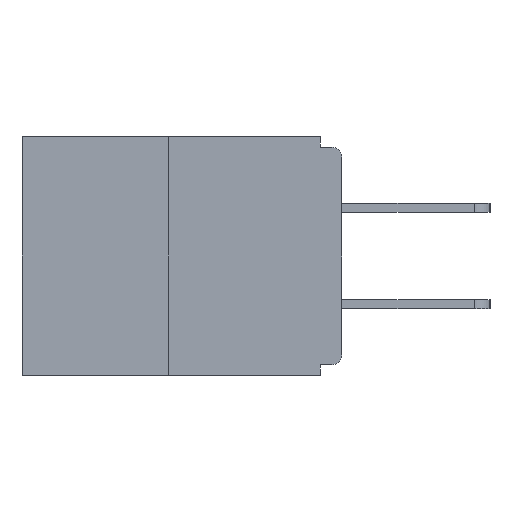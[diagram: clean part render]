
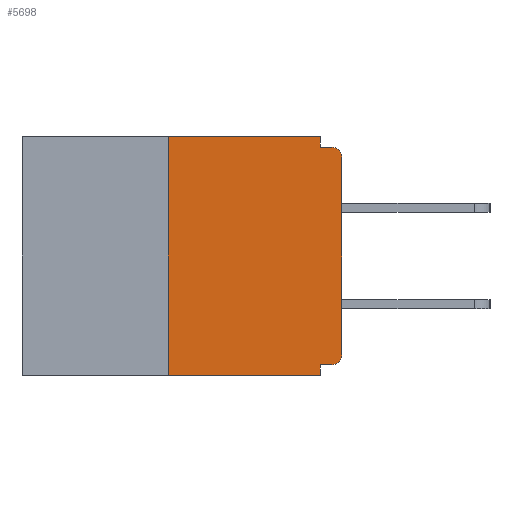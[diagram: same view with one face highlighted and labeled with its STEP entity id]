
A CAD part, left-side view. The second image highlights one B-rep face of the part: STEP entity #5698.
In plain terms, the highlighted planar face has unit normal (-1, 0, 0).
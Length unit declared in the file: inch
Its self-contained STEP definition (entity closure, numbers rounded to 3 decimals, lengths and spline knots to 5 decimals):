
#216 = EDGE_CURVE ( 'NONE', #15936, #7112, #509, .T. ) ;
#248 = LINE ( 'NONE', #10143, #14799 ) ;
#308 = ORIENTED_EDGE ( 'NONE', *, *, #7261, .F. ) ;
#509 = LINE ( 'NONE', #12860, #3932 ) ;
#842 = CARTESIAN_POINT ( 'NONE',  ( 0., 0., -0.328 ) ) ;
#1045 = CARTESIAN_POINT ( 'NONE',  ( 0., 0.031, -0.015 ) ) ;
#1249 = DIRECTION ( 'NONE',  ( 1., 0., 0. ) ) ;
#1310 = AXIS2_PLACEMENT_3D ( 'NONE', #16571, #11235, #15291 ) ;
#1340 = EDGE_LOOP ( 'NONE', ( #10820, #16333, #9954, #6503, #308, #12180, #6165, #7404, #17594, #8028 ) ) ;
#1341 = PLANE ( 'NONE',  #3273 ) ;
#1523 = EDGE_CURVE ( 'NONE', #9903, #10534, #248, .T. ) ;
#1557 = LINE ( 'NONE', #13968, #10172 ) ;
#1688 = LINE ( 'NONE', #14015, #9196 ) ;
#2041 = CARTESIAN_POINT ( 'NONE',  ( 0., 0.015, -0.328 ) ) ;
#2292 = CARTESIAN_POINT ( 'NONE',  ( 0., 0., -0.03 ) ) ;
#2333 = EDGE_CURVE ( 'NONE', #14683, #17802, #9135, .T. ) ;
#2402 = VERTEX_POINT ( 'NONE', #2791 ) ;
#2473 = DIRECTION ( 'NONE',  ( 0., 1., 0. ) ) ;
#2717 = EDGE_CURVE ( 'NONE', #6526, #2402, #1688, .T. ) ;
#2791 = CARTESIAN_POINT ( 'NONE',  ( 0., 0.031, 0. ) ) ;
#2970 = DIRECTION ( 'NONE',  ( 0., -1., 0. ) ) ;
#3224 = EDGE_CURVE ( 'NONE', #6011, #7112, #15330, .T. ) ;
#3273 = AXIS2_PLACEMENT_3D ( 'NONE', #10781, #1249, #9414 ) ;
#3932 = VECTOR ( 'NONE', #2970, 39.37008 ) ;
#4334 = CARTESIAN_POINT ( 'NONE',  ( 0., 0.25, 0. ) ) ;
#5257 = VECTOR ( 'NONE', #14759, 39.37008 ) ;
#5698 = ADVANCED_FACE ( 'NONE', ( #12320 ), #1341, .F. ) ;
#6011 = VERTEX_POINT ( 'NONE', #6547 ) ;
#6165 = ORIENTED_EDGE ( 'NONE', *, *, #7522, .T. ) ;
#6370 = LINE ( 'NONE', #842, #9328 ) ;
#6503 = ORIENTED_EDGE ( 'NONE', *, *, #3224, .F. ) ;
#6526 = VERTEX_POINT ( 'NONE', #4334 ) ;
#6547 = CARTESIAN_POINT ( 'NONE',  ( 0., 0.031, -0.328 ) ) ;
#6829 = CARTESIAN_POINT ( 'NONE',  ( 0., 0.031, -0.343 ) ) ;
#7112 = VERTEX_POINT ( 'NONE', #13197 ) ;
#7261 = EDGE_CURVE ( 'NONE', #14683, #6011, #6370, .T. ) ;
#7404 = ORIENTED_EDGE ( 'NONE', *, *, #12833, .T. ) ;
#7458 = CARTESIAN_POINT ( 'NONE',  ( 0., 0., 0. ) ) ;
#7522 = EDGE_CURVE ( 'NONE', #17802, #17340, #10614, .T. ) ;
#7914 = CARTESIAN_POINT ( 'NONE',  ( 0., 0.031, 0. ) ) ;
#8028 = ORIENTED_EDGE ( 'NONE', *, *, #10274, .F. ) ;
#8495 = DIRECTION ( 'NONE',  ( 0., -1., 0. ) ) ;
#9135 = CIRCLE ( 'NONE', #1310, 0.015 ) ;
#9196 = VECTOR ( 'NONE', #8495, 39.37008 ) ;
#9328 = VECTOR ( 'NONE', #2473, 39.37008 ) ;
#9411 = CARTESIAN_POINT ( 'NONE',  ( 0., 0.015, -0.015 ) ) ;
#9414 = DIRECTION ( 'NONE',  ( 0., 0., -1. ) ) ;
#9874 = CARTESIAN_POINT ( 'NONE',  ( 0., 0.015, -0.03 ) ) ;
#9903 = VERTEX_POINT ( 'NONE', #1045 ) ;
#9954 = ORIENTED_EDGE ( 'NONE', *, *, #216, .T. ) ;
#10143 = CARTESIAN_POINT ( 'NONE',  ( 0., 0., -0.015 ) ) ;
#10145 = AXIS2_PLACEMENT_3D ( 'NONE', #9874, #15030, #10973 ) ;
#10172 = VECTOR ( 'NONE', #12527, 39.37008 ) ;
#10235 = DIRECTION ( 'NONE',  ( 0., -1., 0. ) ) ;
#10274 = EDGE_CURVE ( 'NONE', #2402, #9903, #12169, .T. ) ;
#10534 = VERTEX_POINT ( 'NONE', #9411 ) ;
#10614 = LINE ( 'NONE', #7458, #5257 ) ;
#10727 = DIRECTION ( 'NONE',  ( 0., 0., -1. ) ) ;
#10781 = CARTESIAN_POINT ( 'NONE',  ( 0., 0.46, 0. ) ) ;
#10820 = ORIENTED_EDGE ( 'NONE', *, *, #2717, .F. ) ;
#10973 = DIRECTION ( 'NONE',  ( 0., 0., -1. ) ) ;
#11010 = CIRCLE ( 'NONE', #10145, 0.015 ) ;
#11235 = DIRECTION ( 'NONE',  ( -1., 0., 0. ) ) ;
#12169 = LINE ( 'NONE', #7914, #14970 ) ;
#12180 = ORIENTED_EDGE ( 'NONE', *, *, #2333, .T. ) ;
#12320 = FACE_OUTER_BOUND ( 'NONE', #1340, .T. ) ;
#12527 = DIRECTION ( 'NONE',  ( 0., 0., 1. ) ) ;
#12833 = EDGE_CURVE ( 'NONE', #17340, #10534, #11010, .T. ) ;
#12860 = CARTESIAN_POINT ( 'NONE',  ( 0., 0.46, -0.343 ) ) ;
#13197 = CARTESIAN_POINT ( 'NONE',  ( 0., 0.031, -0.343 ) ) ;
#13692 = EDGE_CURVE ( 'NONE', #15936, #6526, #1557, .T. ) ;
#13968 = CARTESIAN_POINT ( 'NONE',  ( 0., 0.25, 0. ) ) ;
#14015 = CARTESIAN_POINT ( 'NONE',  ( 0., 0.46, 0. ) ) ;
#14683 = VERTEX_POINT ( 'NONE', #2041 ) ;
#14759 = DIRECTION ( 'NONE',  ( 0., 0., 1. ) ) ;
#14799 = VECTOR ( 'NONE', #10235, 39.37008 ) ;
#14970 = VECTOR ( 'NONE', #10727, 39.37008 ) ;
#15030 = DIRECTION ( 'NONE',  ( -1., 0., 0. ) ) ;
#15073 = VECTOR ( 'NONE', #16801, 39.37008 ) ;
#15291 = DIRECTION ( 'NONE',  ( 0., 0., -1. ) ) ;
#15330 = LINE ( 'NONE', #6829, #15073 ) ;
#15571 = CARTESIAN_POINT ( 'NONE',  ( 0., 0.25, -0.343 ) ) ;
#15936 = VERTEX_POINT ( 'NONE', #15571 ) ;
#16333 = ORIENTED_EDGE ( 'NONE', *, *, #13692, .F. ) ;
#16571 = CARTESIAN_POINT ( 'NONE',  ( 0., 0.015, -0.313 ) ) ;
#16801 = DIRECTION ( 'NONE',  ( 0., 0., -1. ) ) ;
#17164 = CARTESIAN_POINT ( 'NONE',  ( 0., 0., -0.313 ) ) ;
#17340 = VERTEX_POINT ( 'NONE', #2292 ) ;
#17594 = ORIENTED_EDGE ( 'NONE', *, *, #1523, .F. ) ;
#17802 = VERTEX_POINT ( 'NONE', #17164 ) ;
